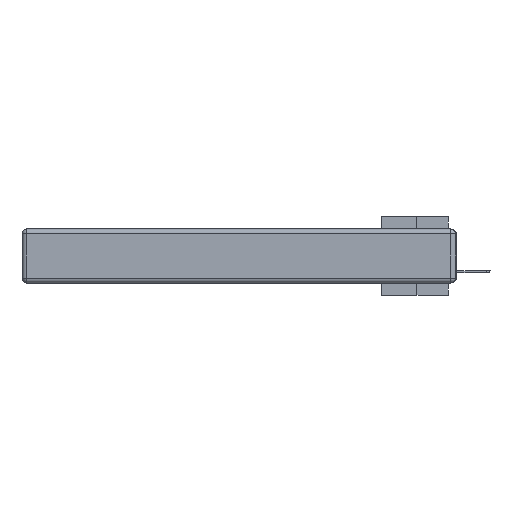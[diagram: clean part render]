
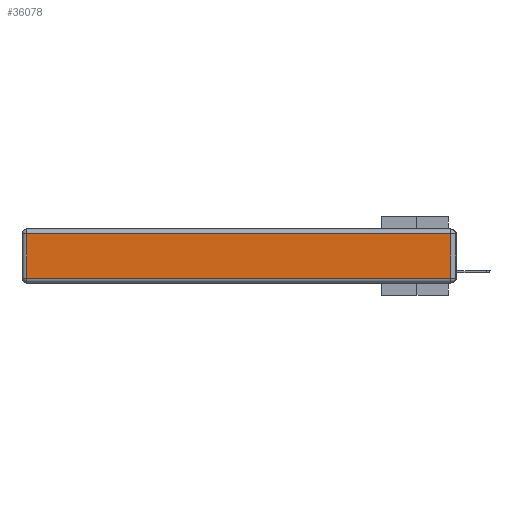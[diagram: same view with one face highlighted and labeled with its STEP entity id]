
A CAD part, left-side view. The second image highlights one B-rep face of the part: STEP entity #36078.
In plain terms, the highlighted planar face has unit normal (-1, 0, 0).
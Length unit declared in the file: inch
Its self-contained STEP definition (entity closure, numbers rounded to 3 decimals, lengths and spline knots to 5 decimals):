
#1855 = LINE ( 'NONE', #25347, #6993 ) ;
#2931 = DIRECTION ( 'NONE',  ( 0., 0., 1. ) ) ;
#4085 = DIRECTION ( 'NONE',  ( 0., 1., 0. ) ) ;
#4277 = CARTESIAN_POINT ( 'NONE',  ( 0., 0., -0.343 ) ) ;
#4993 = CARTESIAN_POINT ( 'NONE',  ( 0., 0.03, -0.313 ) ) ;
#5467 = ORIENTED_EDGE ( 'NONE', *, *, #10168, .T. ) ;
#6413 = VECTOR ( 'NONE', #2931, 39.37008 ) ;
#6993 = VECTOR ( 'NONE', #37034, 39.37008 ) ;
#7281 = LINE ( 'NONE', #15581, #28208 ) ;
#7370 = EDGE_CURVE ( 'NONE', #19147, #8365, #19625, .T. ) ;
#7397 = CARTESIAN_POINT ( 'NONE',  ( 0., 2.72, -0.03 ) ) ;
#8365 = VERTEX_POINT ( 'NONE', #7397 ) ;
#10168 = EDGE_CURVE ( 'NONE', #8365, #37784, #1855, .T. ) ;
#10580 = CARTESIAN_POINT ( 'NONE',  ( 0., 2.72, -0.313 ) ) ;
#11175 = CARTESIAN_POINT ( 'NONE',  ( 0., 0.03, -0.03 ) ) ;
#11211 = ORIENTED_EDGE ( 'NONE', *, *, #33775, .T. ) ;
#11770 = CARTESIAN_POINT ( 'NONE',  ( 0., 0.03, -0.343 ) ) ;
#12296 = EDGE_CURVE ( 'NONE', #37681, #19147, #17564, .T. ) ;
#15581 = CARTESIAN_POINT ( 'NONE',  ( 0., 0., -0.313 ) ) ;
#15656 = DIRECTION ( 'NONE',  ( -1., 0., 0. ) ) ;
#17564 = LINE ( 'NONE', #11770, #6413 ) ;
#19147 = VERTEX_POINT ( 'NONE', #11175 ) ;
#19426 = CARTESIAN_POINT ( 'NONE',  ( 0., 2.75, -0.03 ) ) ;
#19625 = LINE ( 'NONE', #19426, #33832 ) ;
#21436 = FACE_OUTER_BOUND ( 'NONE', #31496, .T. ) ;
#25066 = DIRECTION ( 'NONE',  ( 0., 0., 1. ) ) ;
#25347 = CARTESIAN_POINT ( 'NONE',  ( 0., 2.72, -0.343 ) ) ;
#28208 = VECTOR ( 'NONE', #30943, 39.37008 ) ;
#30462 = PLANE ( 'NONE',  #37551 ) ;
#30943 = DIRECTION ( 'NONE',  ( 0., -1., 0. ) ) ;
#31496 = EDGE_LOOP ( 'NONE', ( #11211, #36079, #33715, #5467 ) ) ;
#33715 = ORIENTED_EDGE ( 'NONE', *, *, #7370, .T. ) ;
#33775 = EDGE_CURVE ( 'NONE', #37784, #37681, #7281, .T. ) ;
#33832 = VECTOR ( 'NONE', #4085, 39.37008 ) ;
#36078 = ADVANCED_FACE ( 'NONE', ( #21436 ), #30462, .T. ) ;
#36079 = ORIENTED_EDGE ( 'NONE', *, *, #12296, .T. ) ;
#37034 = DIRECTION ( 'NONE',  ( 0., 0., -1. ) ) ;
#37551 = AXIS2_PLACEMENT_3D ( 'NONE', #4277, #15656, #25066 ) ;
#37681 = VERTEX_POINT ( 'NONE', #4993 ) ;
#37784 = VERTEX_POINT ( 'NONE', #10580 ) ;
